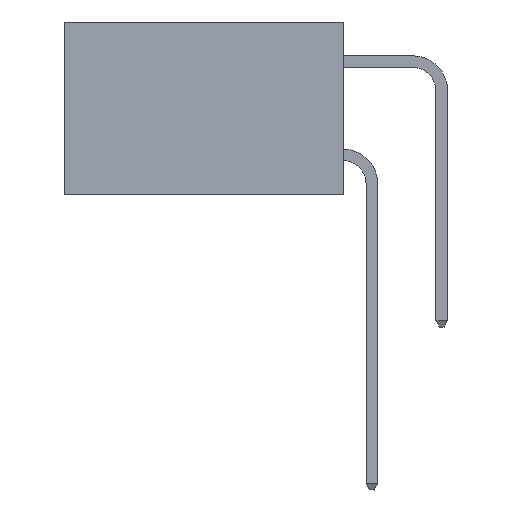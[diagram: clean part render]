
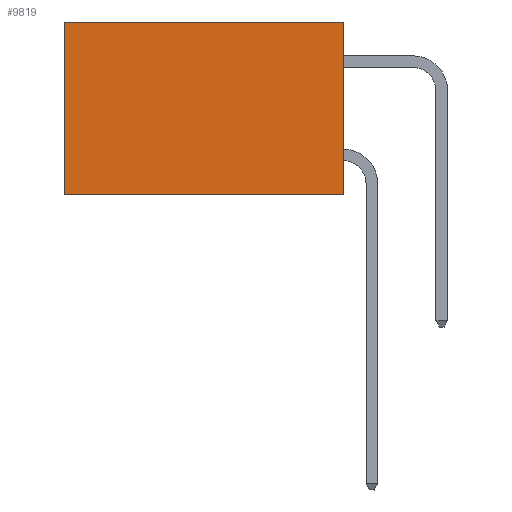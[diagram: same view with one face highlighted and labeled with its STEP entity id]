
A CAD part, left-side view. The second image highlights one B-rep face of the part: STEP entity #9819.
In plain terms, the highlighted planar face has unit normal (-1, 0, 0).
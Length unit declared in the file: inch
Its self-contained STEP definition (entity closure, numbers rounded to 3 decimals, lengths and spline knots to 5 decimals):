
#200 = CARTESIAN_POINT ( 'NONE',  ( 0.298, 0., -0.37 ) ) ;
#445 = EDGE_CURVE ( 'NONE', #7475, #11884, #622, .T. ) ;
#622 = LINE ( 'NONE', #7583, #12463 ) ;
#1227 = CARTESIAN_POINT ( 'NONE',  ( 0.298, 0., 0. ) ) ;
#2009 = VERTEX_POINT ( 'NONE', #5054 ) ;
#2916 = CARTESIAN_POINT ( 'NONE',  ( 0.298, 0., 0. ) ) ;
#3644 = AXIS2_PLACEMENT_3D ( 'NONE', #2916, #13240, #5951 ) ;
#4398 = CARTESIAN_POINT ( 'NONE',  ( 0.298, 0., 0. ) ) ;
#4402 = EDGE_LOOP ( 'NONE', ( #14181, #6173, #16486, #15120 ) ) ;
#5054 = CARTESIAN_POINT ( 'NONE',  ( 0.298, 0.6, -0.37 ) ) ;
#5253 = DIRECTION ( 'NONE',  ( 0., 0., -1. ) ) ;
#5363 = VECTOR ( 'NONE', #11997, 39.37008 ) ;
#5598 = LINE ( 'NONE', #7726, #15319 ) ;
#5818 = PLANE ( 'NONE',  #3644 ) ;
#5951 = DIRECTION ( 'NONE',  ( 0., 0., -1. ) ) ;
#5996 = EDGE_CURVE ( 'NONE', #11884, #2009, #12706, .T. ) ;
#6173 = ORIENTED_EDGE ( 'NONE', *, *, #15686, .F. ) ;
#7475 = VERTEX_POINT ( 'NONE', #1227 ) ;
#7583 = CARTESIAN_POINT ( 'NONE',  ( 0.298, 0., 0. ) ) ;
#7726 = CARTESIAN_POINT ( 'NONE',  ( 0.298, 0., -0.37 ) ) ;
#7837 = DIRECTION ( 'NONE',  ( 0., 1., 0. ) ) ;
#8030 = CARTESIAN_POINT ( 'NONE',  ( 0.298, 0.6, 0. ) ) ;
#8171 = CARTESIAN_POINT ( 'NONE',  ( 0.298, 0.6, 0. ) ) ;
#8759 = VECTOR ( 'NONE', #5253, 39.37008 ) ;
#9819 = ADVANCED_FACE ( 'NONE', ( #14091 ), #5818, .F. ) ;
#11391 = LINE ( 'NONE', #4398, #5363 ) ;
#11771 = VERTEX_POINT ( 'NONE', #200 ) ;
#11884 = VERTEX_POINT ( 'NONE', #8030 ) ;
#11997 = DIRECTION ( 'NONE',  ( 0., 0., -1. ) ) ;
#12234 = DIRECTION ( 'NONE',  ( 0., 1., 0. ) ) ;
#12463 = VECTOR ( 'NONE', #12234, 39.37008 ) ;
#12706 = LINE ( 'NONE', #8171, #8759 ) ;
#13240 = DIRECTION ( 'NONE',  ( 1., 0., 0. ) ) ;
#14091 = FACE_OUTER_BOUND ( 'NONE', #4402, .T. ) ;
#14181 = ORIENTED_EDGE ( 'NONE', *, *, #5996, .T. ) ;
#15120 = ORIENTED_EDGE ( 'NONE', *, *, #445, .T. ) ;
#15226 = EDGE_CURVE ( 'NONE', #7475, #11771, #11391, .T. ) ;
#15319 = VECTOR ( 'NONE', #7837, 39.37008 ) ;
#15686 = EDGE_CURVE ( 'NONE', #11771, #2009, #5598, .T. ) ;
#16486 = ORIENTED_EDGE ( 'NONE', *, *, #15226, .F. ) ;
